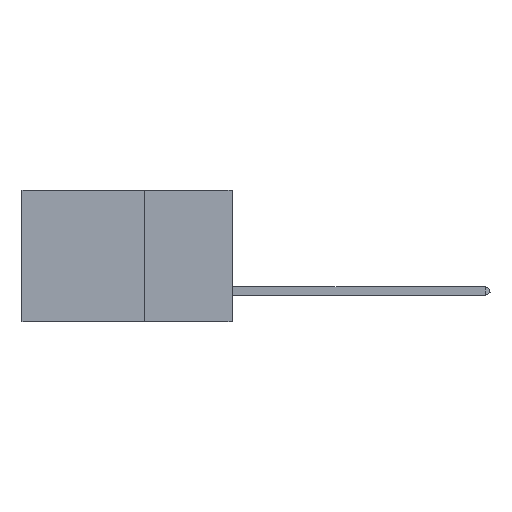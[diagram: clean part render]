
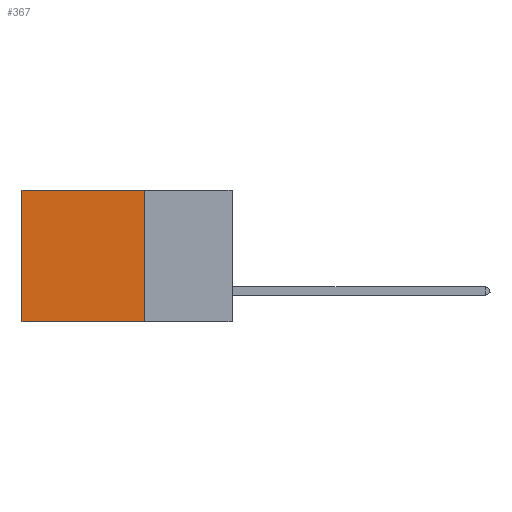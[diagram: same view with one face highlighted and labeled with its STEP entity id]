
A CAD part, left-side view. The second image highlights one B-rep face of the part: STEP entity #367.
In plain terms, the highlighted planar face has unit normal (-1, 0, 0).
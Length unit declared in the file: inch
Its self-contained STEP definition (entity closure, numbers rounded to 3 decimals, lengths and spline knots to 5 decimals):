
#85 = DIRECTION ( 'NONE',  ( 0., 1., 0. ) ) ;
#367 = ADVANCED_FACE ( 'NONE', ( #6147 ), #984, .F. ) ;
#514 = EDGE_CURVE ( 'NONE', #5013, #5847, #7317, .T. ) ;
#732 = VERTEX_POINT ( 'NONE', #7883 ) ;
#887 = VECTOR ( 'NONE', #13514, 39.37008 ) ;
#984 = PLANE ( 'NONE',  #8021 ) ;
#1215 = CARTESIAN_POINT ( 'NONE',  ( 0.2875, 0.25, 0. ) ) ;
#1378 = ORIENTED_EDGE ( 'NONE', *, *, #15042, .T. ) ;
#1611 = ORIENTED_EDGE ( 'NONE', *, *, #11954, .T. ) ;
#2297 = VECTOR ( 'NONE', #5798, 39.37008 ) ;
#3050 = CARTESIAN_POINT ( 'NONE',  ( 0.2875, 0.25, -0.375 ) ) ;
#3087 = LINE ( 'NONE', #11964, #2297 ) ;
#3101 = CARTESIAN_POINT ( 'NONE',  ( 0.2875, 0.25, -0.375 ) ) ;
#3201 = DIRECTION ( 'NONE',  ( 0., 0., -1. ) ) ;
#3377 = DIRECTION ( 'NONE',  ( 1., 0., 0. ) ) ;
#3404 = LINE ( 'NONE', #3050, #11588 ) ;
#4781 = CARTESIAN_POINT ( 'NONE',  ( 0.2875, 0.25, -0.375 ) ) ;
#4846 = CARTESIAN_POINT ( 'NONE',  ( 0.2875, 0.25, -0.375 ) ) ;
#4932 = LINE ( 'NONE', #1215, #11782 ) ;
#5013 = VERTEX_POINT ( 'NONE', #3101 ) ;
#5632 = ORIENTED_EDGE ( 'NONE', *, *, #14721, .F. ) ;
#5798 = DIRECTION ( 'NONE',  ( 0., 0., -1. ) ) ;
#5847 = VERTEX_POINT ( 'NONE', #7422 ) ;
#6147 = FACE_OUTER_BOUND ( 'NONE', #11302, .T. ) ;
#7158 = DIRECTION ( 'NONE',  ( 0., 0., -1. ) ) ;
#7317 = LINE ( 'NONE', #4846, #887 ) ;
#7422 = CARTESIAN_POINT ( 'NONE',  ( 0.2875, 0.6, -0.375 ) ) ;
#7883 = CARTESIAN_POINT ( 'NONE',  ( 0.2875, 0.25, 0. ) ) ;
#8021 = AXIS2_PLACEMENT_3D ( 'NONE', #4781, #3377, #7158 ) ;
#8451 = VERTEX_POINT ( 'NONE', #12017 ) ;
#11302 = EDGE_LOOP ( 'NONE', ( #1611, #15862, #5632, #1378 ) ) ;
#11588 = VECTOR ( 'NONE', #3201, 39.37008 ) ;
#11782 = VECTOR ( 'NONE', #85, 39.37008 ) ;
#11954 = EDGE_CURVE ( 'NONE', #8451, #5847, #3087, .T. ) ;
#11964 = CARTESIAN_POINT ( 'NONE',  ( 0.2875, 0.6, -0.375 ) ) ;
#12017 = CARTESIAN_POINT ( 'NONE',  ( 0.2875, 0.6, 0. ) ) ;
#13514 = DIRECTION ( 'NONE',  ( 0., 1., 0. ) ) ;
#14721 = EDGE_CURVE ( 'NONE', #732, #5013, #3404, .T. ) ;
#15042 = EDGE_CURVE ( 'NONE', #732, #8451, #4932, .T. ) ;
#15862 = ORIENTED_EDGE ( 'NONE', *, *, #514, .F. ) ;
